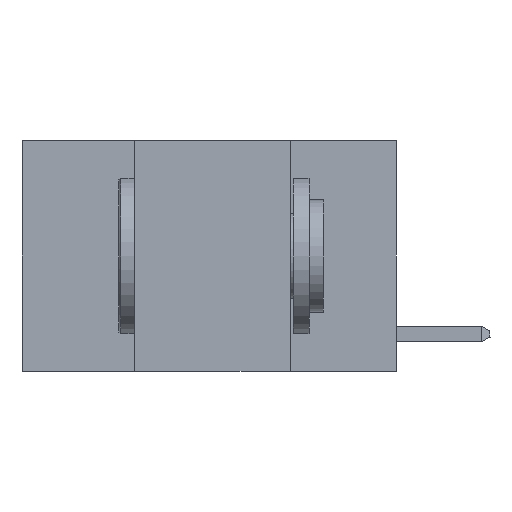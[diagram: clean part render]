
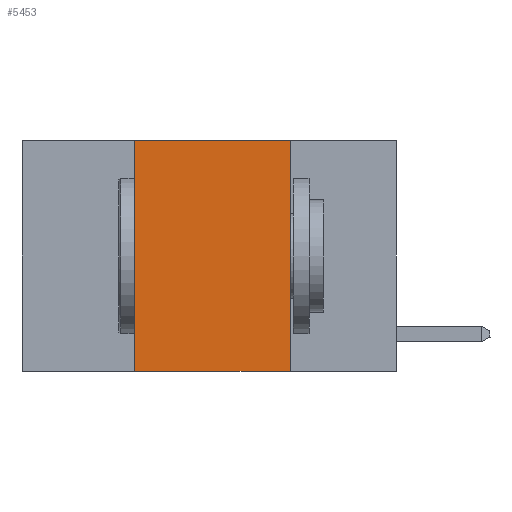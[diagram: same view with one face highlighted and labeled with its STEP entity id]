
A CAD part, left-side view. The second image highlights one B-rep face of the part: STEP entity #5453.
In plain terms, the highlighted planar face has unit normal (-1, 0, 0).
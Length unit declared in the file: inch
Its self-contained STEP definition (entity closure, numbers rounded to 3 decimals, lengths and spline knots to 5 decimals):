
#248 = VERTEX_POINT ( 'NONE', #2393 ) ;
#671 = DIRECTION ( 'NONE',  ( 0., 0., -1. ) ) ;
#1278 = VECTOR ( 'NONE', #9246, 39.37008 ) ;
#1760 = CARTESIAN_POINT ( 'NONE',  ( 0., 0.6, -0.37 ) ) ;
#1909 = EDGE_CURVE ( 'NONE', #10699, #248, #5777, .T. ) ;
#2180 = EDGE_CURVE ( 'NONE', #10699, #11815, #3022, .T. ) ;
#2393 = CARTESIAN_POINT ( 'NONE',  ( 0., 0.42, 0. ) ) ;
#3022 = LINE ( 'NONE', #1760, #1278 ) ;
#3425 = EDGE_LOOP ( 'NONE', ( #11981, #14611, #3496, #12356 ) ) ;
#3463 = EDGE_CURVE ( 'NONE', #248, #6304, #15975, .T. ) ;
#3496 = ORIENTED_EDGE ( 'NONE', *, *, #1909, .F. ) ;
#3578 = VECTOR ( 'NONE', #15096, 39.37008 ) ;
#3856 = LINE ( 'NONE', #6418, #3578 ) ;
#4115 = PLANE ( 'NONE',  #8984 ) ;
#5312 = CARTESIAN_POINT ( 'NONE',  ( 0., 0.6, 0. ) ) ;
#5453 = ADVANCED_FACE ( 'NONE', ( #13156 ), #4115, .F. ) ;
#5777 = LINE ( 'NONE', #14609, #13429 ) ;
#5961 = EDGE_CURVE ( 'NONE', #6304, #11815, #3856, .T. ) ;
#5993 = DIRECTION ( 'NONE',  ( 0., -1., 0. ) ) ;
#6304 = VERTEX_POINT ( 'NONE', #11007 ) ;
#6418 = CARTESIAN_POINT ( 'NONE',  ( 0., 0.17, 0. ) ) ;
#8543 = CARTESIAN_POINT ( 'NONE',  ( 0., 0.42, -0.37 ) ) ;
#8984 = AXIS2_PLACEMENT_3D ( 'NONE', #5312, #10292, #671 ) ;
#9246 = DIRECTION ( 'NONE',  ( 0., -1., 0. ) ) ;
#9527 = VECTOR ( 'NONE', #5993, 39.37008 ) ;
#10292 = DIRECTION ( 'NONE',  ( 1., 0., 0. ) ) ;
#10699 = VERTEX_POINT ( 'NONE', #8543 ) ;
#11007 = CARTESIAN_POINT ( 'NONE',  ( 0., 0.17, 0. ) ) ;
#11815 = VERTEX_POINT ( 'NONE', #12143 ) ;
#11981 = ORIENTED_EDGE ( 'NONE', *, *, #5961, .F. ) ;
#12143 = CARTESIAN_POINT ( 'NONE',  ( 0., 0.17, -0.37 ) ) ;
#12356 = ORIENTED_EDGE ( 'NONE', *, *, #2180, .T. ) ;
#13156 = FACE_OUTER_BOUND ( 'NONE', #3425, .T. ) ;
#13429 = VECTOR ( 'NONE', #15759, 39.37008 ) ;
#14609 = CARTESIAN_POINT ( 'NONE',  ( 0., 0.42, 0. ) ) ;
#14611 = ORIENTED_EDGE ( 'NONE', *, *, #3463, .F. ) ;
#14663 = CARTESIAN_POINT ( 'NONE',  ( 0., 0.6, 0. ) ) ;
#15096 = DIRECTION ( 'NONE',  ( 0., 0., -1. ) ) ;
#15759 = DIRECTION ( 'NONE',  ( 0., 0., 1. ) ) ;
#15975 = LINE ( 'NONE', #14663, #9527 ) ;
